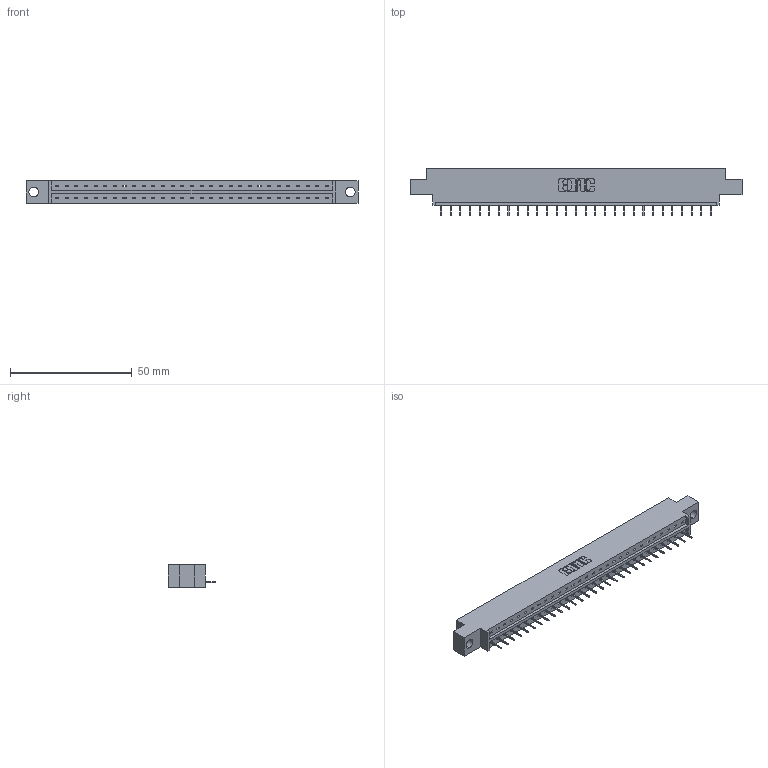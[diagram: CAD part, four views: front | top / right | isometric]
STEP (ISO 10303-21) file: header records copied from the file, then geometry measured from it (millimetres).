
FILE_DESCRIPTION (( 'STEP AP203' ), '1' );
FILE_NAME ('333-029-524-604.STEP', '2018-08-02T16:26:51', ( '' ), ( '' ), 'SwSTEP 2.0', 'SolidWorks 2016', '' );
FILE_SCHEMA (( 'CONFIG_CONTROL_DESIGN' ));
Length unit declared in the file: inch
Products named in the file (3): 333 Part_Offset - .156 Dia - TH; 345-292-001_345-293-124; 333-029-524-604
Assembly tree (30 placements, depth 2):
  333-029-524-604
    333 Part_Offset - .156 Dia - TH
    345-292-001_345-293-124  x29
Bounding box: 136.45 x 19.69 x 9.4 mm (x, y, z)
Volume: 13188.6 mm3; surface area: 13784.4 mm2
Topology: 30 solids, 30 shells, 1916 faces, 5543 edges, 3578 vertices
Faces by surface type: plane 1466, cylinder 450
Entity records: 19619 total; most frequent: CARTESIAN_POINT 3393, ORIENTED_EDGE 3358, DIRECTION 2889, EDGE_CURVE 1679, LINE 1555, VECTOR 1555, VERTEX_POINT 1114, AXIS2_PLACEMENT_3D 667
